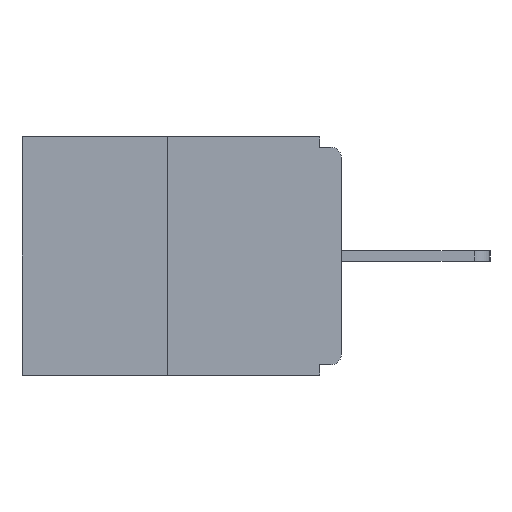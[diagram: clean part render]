
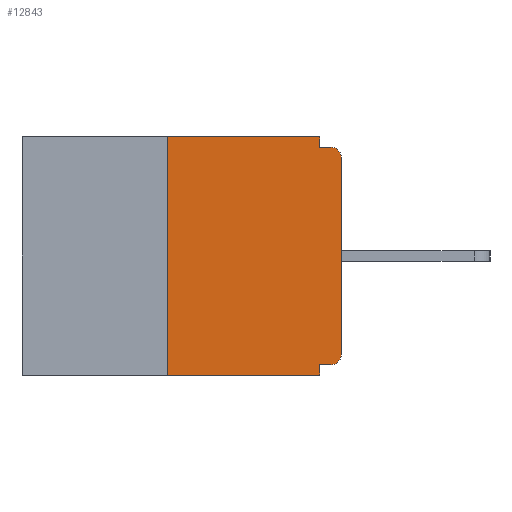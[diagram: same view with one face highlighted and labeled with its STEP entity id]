
A CAD part, left-side view. The second image highlights one B-rep face of the part: STEP entity #12843.
In plain terms, the highlighted planar face has unit normal (-1, 0, 0).
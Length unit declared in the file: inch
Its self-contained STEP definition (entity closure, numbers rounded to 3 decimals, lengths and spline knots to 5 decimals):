
#94 = CARTESIAN_POINT ( 'NONE',  ( 0., 0.46, 0. ) ) ;
#127 = DIRECTION ( 'NONE',  ( 0., 0., -1. ) ) ;
#342 = VECTOR ( 'NONE', #23462, 39.37008 ) ;
#891 = VECTOR ( 'NONE', #8893, 39.37008 ) ;
#922 = VECTOR ( 'NONE', #20035, 39.37008 ) ;
#1158 = ORIENTED_EDGE ( 'NONE', *, *, #4180, .T. ) ;
#1618 = CIRCLE ( 'NONE', #15068, 0.015 ) ;
#1764 = DIRECTION ( 'NONE',  ( 0., -1., 0. ) ) ;
#2028 = LINE ( 'NONE', #6461, #3378 ) ;
#2061 = ORIENTED_EDGE ( 'NONE', *, *, #19937, .F. ) ;
#2117 = VECTOR ( 'NONE', #20172, 39.37008 ) ;
#2212 = DIRECTION ( 'NONE',  ( -1., 0., 0. ) ) ;
#2289 = ORIENTED_EDGE ( 'NONE', *, *, #19929, .F. ) ;
#2451 = ORIENTED_EDGE ( 'NONE', *, *, #8918, .F. ) ;
#2814 = CARTESIAN_POINT ( 'NONE',  ( 0., 0.031, -0.328 ) ) ;
#3313 = EDGE_CURVE ( 'NONE', #8184, #15507, #1618, .T. ) ;
#3378 = VECTOR ( 'NONE', #20810, 39.37008 ) ;
#3646 = CARTESIAN_POINT ( 'NONE',  ( 0., 0.46, 0. ) ) ;
#3679 = VERTEX_POINT ( 'NONE', #12615 ) ;
#4147 = LINE ( 'NONE', #6063, #13845 ) ;
#4175 = ORIENTED_EDGE ( 'NONE', *, *, #3313, .T. ) ;
#4180 = EDGE_CURVE ( 'NONE', #15507, #3679, #22226, .T. ) ;
#4377 = DIRECTION ( 'NONE',  ( 1., 0., 0. ) ) ;
#4403 = ORIENTED_EDGE ( 'NONE', *, *, #24437, .T. ) ;
#4598 = CARTESIAN_POINT ( 'NONE',  ( 0., 0., -0.313 ) ) ;
#4719 = CARTESIAN_POINT ( 'NONE',  ( 0., 0.015, -0.313 ) ) ;
#5198 = ORIENTED_EDGE ( 'NONE', *, *, #23602, .F. ) ;
#5397 = CARTESIAN_POINT ( 'NONE',  ( 0., 0.25, -0.343 ) ) ;
#5779 = ORIENTED_EDGE ( 'NONE', *, *, #21417, .F. ) ;
#6063 = CARTESIAN_POINT ( 'NONE',  ( 0., 0.46, -0.343 ) ) ;
#6461 = CARTESIAN_POINT ( 'NONE',  ( 0., 0., -0.328 ) ) ;
#7937 = CARTESIAN_POINT ( 'NONE',  ( 0., 0.25, 0. ) ) ;
#8020 = AXIS2_PLACEMENT_3D ( 'NONE', #14640, #2212, #16741 ) ;
#8184 = VERTEX_POINT ( 'NONE', #26693 ) ;
#8824 = CARTESIAN_POINT ( 'NONE',  ( 0., 0.015, -0.015 ) ) ;
#8833 = CARTESIAN_POINT ( 'NONE',  ( 0., 0., 0. ) ) ;
#8893 = DIRECTION ( 'NONE',  ( 0., 0., 1. ) ) ;
#8918 = EDGE_CURVE ( 'NONE', #14322, #24537, #22345, .T. ) ;
#9813 = EDGE_CURVE ( 'NONE', #26040, #14322, #16273, .T. ) ;
#10149 = CARTESIAN_POINT ( 'NONE',  ( 0., 0.031, -0.343 ) ) ;
#10573 = PLANE ( 'NONE',  #11974 ) ;
#10811 = VECTOR ( 'NONE', #21591, 39.37008 ) ;
#10925 = CARTESIAN_POINT ( 'NONE',  ( 0., 0.031, 0. ) ) ;
#11598 = ORIENTED_EDGE ( 'NONE', *, *, #9813, .F. ) ;
#11974 = AXIS2_PLACEMENT_3D ( 'NONE', #94, #4377, #18825 ) ;
#12615 = CARTESIAN_POINT ( 'NONE',  ( 0., 0., -0.03 ) ) ;
#12843 = ADVANCED_FACE ( 'NONE', ( #13438 ), #10573, .F. ) ;
#13204 = DIRECTION ( 'NONE',  ( 0., 0., -1. ) ) ;
#13438 = FACE_OUTER_BOUND ( 'NONE', #24395, .T. ) ;
#13845 = VECTOR ( 'NONE', #1764, 39.37008 ) ;
#14322 = VERTEX_POINT ( 'NONE', #15065 ) ;
#14640 = CARTESIAN_POINT ( 'NONE',  ( 0., 0.015, -0.03 ) ) ;
#15065 = CARTESIAN_POINT ( 'NONE',  ( 0., 0.031, -0.015 ) ) ;
#15068 = AXIS2_PLACEMENT_3D ( 'NONE', #4719, #15657, #13204 ) ;
#15072 = CIRCLE ( 'NONE', #8020, 0.015 ) ;
#15226 = VERTEX_POINT ( 'NONE', #7937 ) ;
#15507 = VERTEX_POINT ( 'NONE', #4598 ) ;
#15657 = DIRECTION ( 'NONE',  ( -1., 0., 0. ) ) ;
#16273 = LINE ( 'NONE', #21963, #10811 ) ;
#16719 = CARTESIAN_POINT ( 'NONE',  ( 0., 0.031, -0.343 ) ) ;
#16741 = DIRECTION ( 'NONE',  ( 0., 0., -1. ) ) ;
#16989 = VERTEX_POINT ( 'NONE', #2814 ) ;
#17361 = EDGE_CURVE ( 'NONE', #20815, #25212, #4147, .T. ) ;
#17534 = LINE ( 'NONE', #17987, #922 ) ;
#17987 = CARTESIAN_POINT ( 'NONE',  ( 0., 0.25, 0. ) ) ;
#18825 = DIRECTION ( 'NONE',  ( 0., 0., -1. ) ) ;
#19929 = EDGE_CURVE ( 'NONE', #8184, #16989, #2028, .T. ) ;
#19937 = EDGE_CURVE ( 'NONE', #16989, #25212, #23295, .T. ) ;
#20035 = DIRECTION ( 'NONE',  ( 0., 0., 1. ) ) ;
#20172 = DIRECTION ( 'NONE',  ( 0., -1., 0. ) ) ;
#20810 = DIRECTION ( 'NONE',  ( 0., 1., 0. ) ) ;
#20815 = VERTEX_POINT ( 'NONE', #5397 ) ;
#21417 = EDGE_CURVE ( 'NONE', #20815, #15226, #17534, .T. ) ;
#21591 = DIRECTION ( 'NONE',  ( 0., 0., -1. ) ) ;
#21963 = CARTESIAN_POINT ( 'NONE',  ( 0., 0.031, 0. ) ) ;
#22226 = LINE ( 'NONE', #8833, #891 ) ;
#22345 = LINE ( 'NONE', #23580, #342 ) ;
#23295 = LINE ( 'NONE', #16719, #24549 ) ;
#23462 = DIRECTION ( 'NONE',  ( 0., -1., 0. ) ) ;
#23580 = CARTESIAN_POINT ( 'NONE',  ( 0., 0., -0.015 ) ) ;
#23602 = EDGE_CURVE ( 'NONE', #15226, #26040, #23991, .T. ) ;
#23758 = ORIENTED_EDGE ( 'NONE', *, *, #17361, .T. ) ;
#23991 = LINE ( 'NONE', #3646, #2117 ) ;
#24395 = EDGE_LOOP ( 'NONE', ( #5198, #5779, #23758, #2061, #2289, #4175, #1158, #4403, #2451, #11598 ) ) ;
#24437 = EDGE_CURVE ( 'NONE', #3679, #24537, #15072, .T. ) ;
#24537 = VERTEX_POINT ( 'NONE', #8824 ) ;
#24549 = VECTOR ( 'NONE', #127, 39.37008 ) ;
#25212 = VERTEX_POINT ( 'NONE', #10149 ) ;
#26040 = VERTEX_POINT ( 'NONE', #10925 ) ;
#26693 = CARTESIAN_POINT ( 'NONE',  ( 0., 0.015, -0.328 ) ) ;
